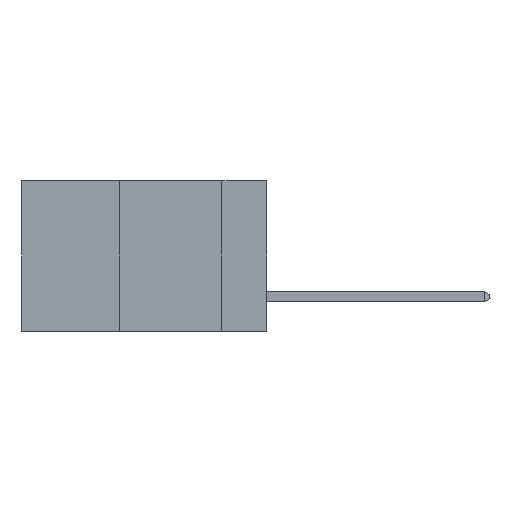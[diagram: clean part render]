
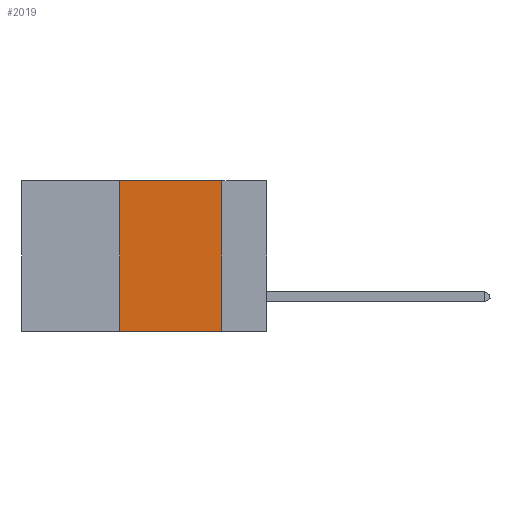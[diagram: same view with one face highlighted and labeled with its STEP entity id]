
A CAD part, left-side view. The second image highlights one B-rep face of the part: STEP entity #2019.
In plain terms, the highlighted planar face has unit normal (-1, 0, 0).
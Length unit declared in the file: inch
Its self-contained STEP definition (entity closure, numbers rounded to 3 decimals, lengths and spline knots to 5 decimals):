
#147 = CARTESIAN_POINT ( 'NONE',  ( 0., 0.6, 0. ) ) ;
#285 = CARTESIAN_POINT ( 'NONE',  ( 0., 0.11, -0.37 ) ) ;
#399 = LINE ( 'NONE', #147, #3817 ) ;
#749 = ORIENTED_EDGE ( 'NONE', *, *, #1652, .F. ) ;
#1640 = CARTESIAN_POINT ( 'NONE',  ( 0., 0.11, 0. ) ) ;
#1652 = EDGE_CURVE ( 'NONE', #15280, #13887, #7293, .T. ) ;
#2019 = ADVANCED_FACE ( 'NONE', ( #15904 ), #6843, .F. ) ;
#2967 = ORIENTED_EDGE ( 'NONE', *, *, #10493, .F. ) ;
#2986 = VERTEX_POINT ( 'NONE', #18522 ) ;
#3439 = VECTOR ( 'NONE', #6198, 39.37008 ) ;
#3538 = CARTESIAN_POINT ( 'NONE',  ( 0., 0.36, 0. ) ) ;
#3804 = CARTESIAN_POINT ( 'NONE',  ( 0., 0.36, 0. ) ) ;
#3817 = VECTOR ( 'NONE', #11634, 39.37008 ) ;
#3829 = DIRECTION ( 'NONE',  ( 0., 0., 1. ) ) ;
#4225 = DIRECTION ( 'NONE',  ( 1., 0., 0. ) ) ;
#4715 = EDGE_LOOP ( 'NONE', ( #749, #9076, #2967, #9929 ) ) ;
#4872 = EDGE_CURVE ( 'NONE', #2986, #13887, #15091, .T. ) ;
#5432 = DIRECTION ( 'NONE',  ( 0., 0., -1. ) ) ;
#6198 = DIRECTION ( 'NONE',  ( 0., 0., -1. ) ) ;
#6843 = PLANE ( 'NONE',  #8016 ) ;
#7293 = LINE ( 'NONE', #1640, #3439 ) ;
#7838 = VECTOR ( 'NONE', #8427, 39.37008 ) ;
#8016 = AXIS2_PLACEMENT_3D ( 'NONE', #16977, #4225, #5432 ) ;
#8365 = VERTEX_POINT ( 'NONE', #3804 ) ;
#8427 = DIRECTION ( 'NONE',  ( 0., -1., 0. ) ) ;
#8467 = LINE ( 'NONE', #3538, #9139 ) ;
#9076 = ORIENTED_EDGE ( 'NONE', *, *, #14807, .F. ) ;
#9139 = VECTOR ( 'NONE', #3829, 39.37008 ) ;
#9929 = ORIENTED_EDGE ( 'NONE', *, *, #4872, .T. ) ;
#10493 = EDGE_CURVE ( 'NONE', #2986, #8365, #8467, .T. ) ;
#10544 = CARTESIAN_POINT ( 'NONE',  ( 0., 0.11, 0. ) ) ;
#11634 = DIRECTION ( 'NONE',  ( 0., -1., 0. ) ) ;
#13887 = VERTEX_POINT ( 'NONE', #285 ) ;
#14807 = EDGE_CURVE ( 'NONE', #8365, #15280, #399, .T. ) ;
#15091 = LINE ( 'NONE', #15463, #7838 ) ;
#15280 = VERTEX_POINT ( 'NONE', #10544 ) ;
#15463 = CARTESIAN_POINT ( 'NONE',  ( 0., 0.6, -0.37 ) ) ;
#15904 = FACE_OUTER_BOUND ( 'NONE', #4715, .T. ) ;
#16977 = CARTESIAN_POINT ( 'NONE',  ( 0., 0.6, 0. ) ) ;
#18522 = CARTESIAN_POINT ( 'NONE',  ( 0., 0.36, -0.37 ) ) ;
